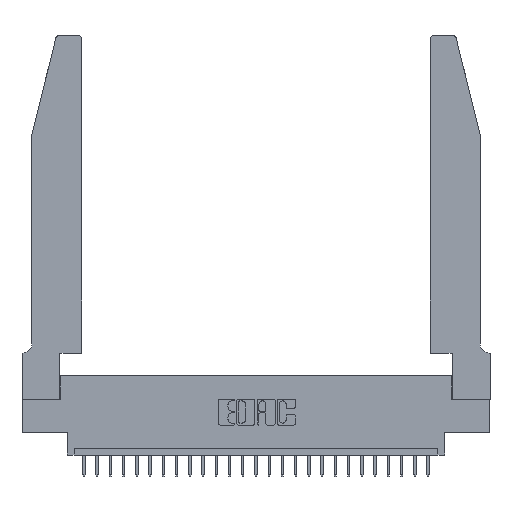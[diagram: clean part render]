
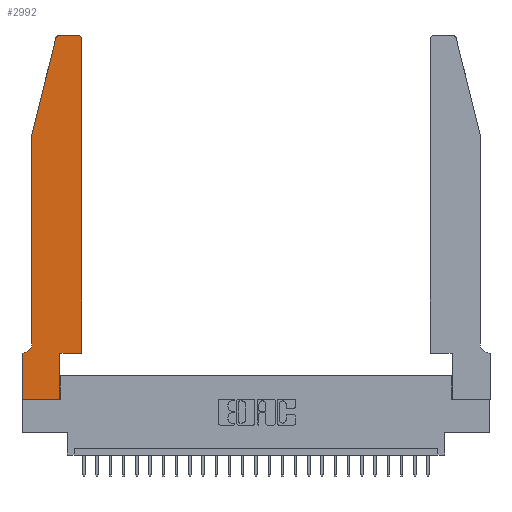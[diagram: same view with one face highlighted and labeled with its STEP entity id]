
A CAD part, top view. The second image highlights one B-rep face of the part: STEP entity #2992.
In plain terms, the highlighted planar face has unit normal (0, 0, 1).
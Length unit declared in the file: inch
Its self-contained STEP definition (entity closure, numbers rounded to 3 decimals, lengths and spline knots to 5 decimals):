
#93 = CARTESIAN_POINT ( 'NONE',  ( 0.2865, 0.35, 0.37 ) ) ;
#133 = CIRCLE ( 'NONE', #20253, 0.07 ) ;
#501 = ORIENTED_EDGE ( 'NONE', *, *, #2947, .T. ) ;
#840 = ORIENTED_EDGE ( 'NONE', *, *, #14292, .T. ) ;
#1494 = VERTEX_POINT ( 'NONE', #27087 ) ;
#1596 = VERTEX_POINT ( 'NONE', #18444 ) ;
#1623 = ORIENTED_EDGE ( 'NONE', *, *, #11877, .T. ) ;
#1687 = DIRECTION ( 'NONE',  ( -1., 0., 0. ) ) ;
#1754 = CARTESIAN_POINT ( 'NONE',  ( 0.284, 2.75, 0.37 ) ) ;
#2171 = VERTEX_POINT ( 'NONE', #13804 ) ;
#2495 = CARTESIAN_POINT ( 'NONE',  ( 0.4505, 2.72, 0.37 ) ) ;
#2943 = PLANE ( 'NONE',  #19488 ) ;
#2947 = EDGE_CURVE ( 'NONE', #1596, #12378, #3610, .T. ) ;
#2992 = ADVANCED_FACE ( 'NONE', ( #18440 ), #2943, .T. ) ;
#3480 = CARTESIAN_POINT ( 'NONE',  ( 0., 0., 0.37 ) ) ;
#3610 = LINE ( 'NONE', #19313, #25326 ) ;
#4125 = VERTEX_POINT ( 'NONE', #2495 ) ;
#4558 = CARTESIAN_POINT ( 'NONE',  ( 0.2865, 0.35, 0.37 ) ) ;
#4560 = DIRECTION ( 'NONE',  ( 1., 0., 0. ) ) ;
#4741 = CARTESIAN_POINT ( 'NONE',  ( 0.4205, 2.72, 0.37 ) ) ;
#6176 = CIRCLE ( 'NONE', #6752, 0.03 ) ;
#6752 = AXIS2_PLACEMENT_3D ( 'NONE', #17732, #13364, #13268 ) ;
#7182 = DIRECTION ( 'NONE',  ( 1., 0., 0. ) ) ;
#7294 = ORIENTED_EDGE ( 'NONE', *, *, #16239, .T. ) ;
#7501 = VECTOR ( 'NONE', #13857, 39.37008 ) ;
#7641 = ORIENTED_EDGE ( 'NONE', *, *, #19886, .T. ) ;
#7848 = CARTESIAN_POINT ( 'NONE',  ( 0.0755, 0.42, 0.37 ) ) ;
#8379 = CARTESIAN_POINT ( 'NONE',  ( 0.2865, 0., 0.37 ) ) ;
#8826 = EDGE_CURVE ( 'NONE', #22750, #17190, #10625, .T. ) ;
#8968 = DIRECTION ( 'NONE',  ( 0., 1., 0. ) ) ;
#9286 = VERTEX_POINT ( 'NONE', #8379 ) ;
#9726 = CIRCLE ( 'NONE', #25163, 0.03 ) ;
#10049 = VECTOR ( 'NONE', #17054, 39.37008 ) ;
#10080 = EDGE_CURVE ( 'NONE', #12378, #2171, #6176, .T. ) ;
#10625 = LINE ( 'NONE', #11318, #19206 ) ;
#10799 = CARTESIAN_POINT ( 'NONE',  ( 0.0755, 2., 0.37 ) ) ;
#11318 = CARTESIAN_POINT ( 'NONE',  ( 0.4505, 0.35, 0.37 ) ) ;
#11842 = ORIENTED_EDGE ( 'NONE', *, *, #8826, .T. ) ;
#11877 = EDGE_CURVE ( 'NONE', #21217, #18080, #15251, .T. ) ;
#12378 = VERTEX_POINT ( 'NONE', #1754 ) ;
#13268 = DIRECTION ( 'NONE',  ( 1., 0., 0. ) ) ;
#13364 = DIRECTION ( 'NONE',  ( 0., 0., 1. ) ) ;
#13655 = LINE ( 'NONE', #16117, #23885 ) ;
#13804 = CARTESIAN_POINT ( 'NONE',  ( 0.25487, 2.72718, 0.37 ) ) ;
#13857 = DIRECTION ( 'NONE',  ( 0., -1., 0. ) ) ;
#14138 = CARTESIAN_POINT ( 'NONE',  ( 0.0055, 0.35, 0.37 ) ) ;
#14292 = EDGE_CURVE ( 'NONE', #9286, #22750, #22083, .T. ) ;
#14438 = VECTOR ( 'NONE', #17229, 39.37008 ) ;
#14509 = ORIENTED_EDGE ( 'NONE', *, *, #26676, .T. ) ;
#14661 = CARTESIAN_POINT ( 'NONE',  ( 0., 0., 0.37 ) ) ;
#15101 = DIRECTION ( 'NONE',  ( 1., 0., 0. ) ) ;
#15140 = DIRECTION ( 'NONE',  ( 0., 0., 1. ) ) ;
#15251 = LINE ( 'NONE', #21271, #15569 ) ;
#15569 = VECTOR ( 'NONE', #21181, 39.37008 ) ;
#15624 = LINE ( 'NONE', #14661, #10049 ) ;
#15752 = LINE ( 'NONE', #21284, #14438 ) ;
#16117 = CARTESIAN_POINT ( 'NONE',  ( 0.0755, 0.35, 0.37 ) ) ;
#16121 = EDGE_CURVE ( 'NONE', #2171, #21217, #15752, .T. ) ;
#16239 = EDGE_CURVE ( 'NONE', #17190, #4125, #25967, .T. ) ;
#16248 = ORIENTED_EDGE ( 'NONE', *, *, #19358, .T. ) ;
#16905 = VERTEX_POINT ( 'NONE', #14138 ) ;
#17054 = DIRECTION ( 'NONE',  ( 1., 0., 0. ) ) ;
#17171 = EDGE_LOOP ( 'NONE', ( #501, #23236, #18789, #1623, #24219, #19509, #14509, #7641, #840, #11842, #7294, #16248 ) ) ;
#17190 = VERTEX_POINT ( 'NONE', #22302 ) ;
#17229 = DIRECTION ( 'NONE',  ( -0.239, -0.971, 0. ) ) ;
#17512 = CARTESIAN_POINT ( 'NONE',  ( 0.4505, 0.35, 0.37 ) ) ;
#17568 = CARTESIAN_POINT ( 'NONE',  ( 0., 0.35, 0.37 ) ) ;
#17732 = CARTESIAN_POINT ( 'NONE',  ( 0.284, 2.72, 0.37 ) ) ;
#18044 = CARTESIAN_POINT ( 'NONE',  ( 0.0055, 0.42, 0.37 ) ) ;
#18080 = VERTEX_POINT ( 'NONE', #7848 ) ;
#18440 = FACE_OUTER_BOUND ( 'NONE', #17171, .T. ) ;
#18444 = CARTESIAN_POINT ( 'NONE',  ( 0.4205, 2.75, 0.37 ) ) ;
#18711 = LINE ( 'NONE', #3480, #7501 ) ;
#18789 = ORIENTED_EDGE ( 'NONE', *, *, #16121, .T. ) ;
#19206 = VECTOR ( 'NONE', #15101, 39.37008 ) ;
#19313 = CARTESIAN_POINT ( 'NONE',  ( 0.2605, 2.75, 0.37 ) ) ;
#19358 = EDGE_CURVE ( 'NONE', #4125, #1596, #9726, .T. ) ;
#19488 = AXIS2_PLACEMENT_3D ( 'NONE', #17568, #19709, #7182 ) ;
#19509 = ORIENTED_EDGE ( 'NONE', *, *, #20331, .T. ) ;
#19709 = DIRECTION ( 'NONE',  ( 0., 0., 1. ) ) ;
#19886 = EDGE_CURVE ( 'NONE', #1494, #9286, #15624, .T. ) ;
#19994 = CARTESIAN_POINT ( 'NONE',  ( 0., 0.35, 0.37 ) ) ;
#20253 = AXIS2_PLACEMENT_3D ( 'NONE', #18044, #21982, #22069 ) ;
#20331 = EDGE_CURVE ( 'NONE', #16905, #27076, #13655, .T. ) ;
#20843 = EDGE_CURVE ( 'NONE', #18080, #16905, #133, .T. ) ;
#21089 = VECTOR ( 'NONE', #8968, 39.37008 ) ;
#21181 = DIRECTION ( 'NONE',  ( 0., -1., 0. ) ) ;
#21217 = VERTEX_POINT ( 'NONE', #10799 ) ;
#21271 = CARTESIAN_POINT ( 'NONE',  ( 0.0755, 2., 0.37 ) ) ;
#21284 = CARTESIAN_POINT ( 'NONE',  ( 0.0755, 2., 0.37 ) ) ;
#21681 = VECTOR ( 'NONE', #26159, 39.37008 ) ;
#21982 = DIRECTION ( 'NONE',  ( 0., 0., -1. ) ) ;
#22069 = DIRECTION ( 'NONE',  ( -1., 0., 0. ) ) ;
#22083 = LINE ( 'NONE', #4558, #21089 ) ;
#22302 = CARTESIAN_POINT ( 'NONE',  ( 0.4505, 0.35, 0.37 ) ) ;
#22750 = VERTEX_POINT ( 'NONE', #93 ) ;
#23236 = ORIENTED_EDGE ( 'NONE', *, *, #10080, .T. ) ;
#23501 = DIRECTION ( 'NONE',  ( -1., 0., 0. ) ) ;
#23885 = VECTOR ( 'NONE', #1687, 39.37008 ) ;
#24219 = ORIENTED_EDGE ( 'NONE', *, *, #20843, .T. ) ;
#25163 = AXIS2_PLACEMENT_3D ( 'NONE', #4741, #15140, #4560 ) ;
#25326 = VECTOR ( 'NONE', #23501, 39.37008 ) ;
#25967 = LINE ( 'NONE', #17512, #21681 ) ;
#26159 = DIRECTION ( 'NONE',  ( 0., 1., 0. ) ) ;
#26676 = EDGE_CURVE ( 'NONE', #27076, #1494, #18711, .T. ) ;
#27076 = VERTEX_POINT ( 'NONE', #19994 ) ;
#27087 = CARTESIAN_POINT ( 'NONE',  ( 0., 0., 0.37 ) ) ;
